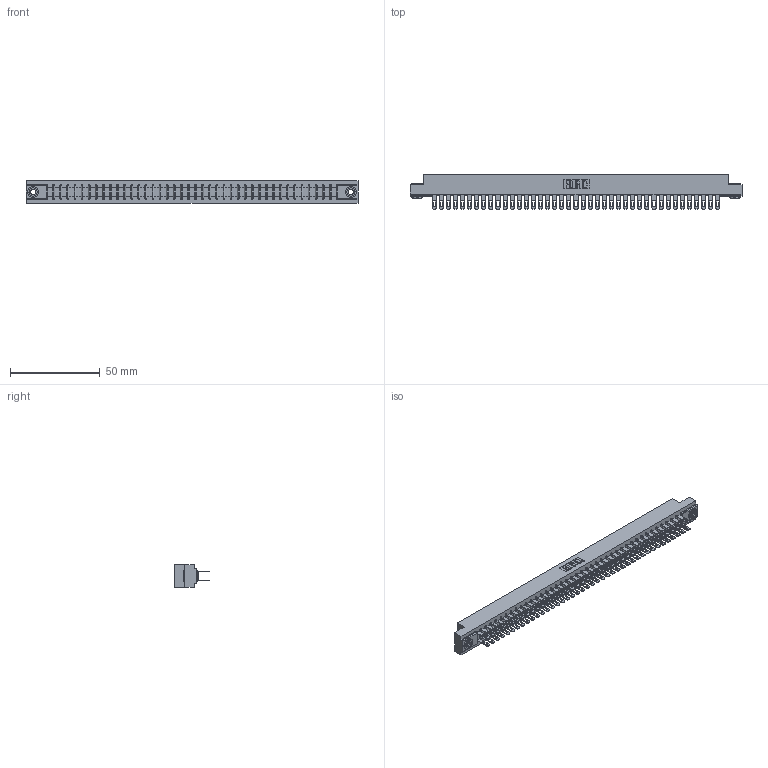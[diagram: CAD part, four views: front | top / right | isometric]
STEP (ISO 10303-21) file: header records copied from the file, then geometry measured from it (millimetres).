
FILE_DESCRIPTION (( 'STEP AP203' ), '1' );
FILE_NAME ('357-082-500-203.STEP', '2018-08-13T00:00:20', ( '' ), ( '' ), 'SwSTEP 2.0', 'SolidWorks 2016', '' );
FILE_SCHEMA (( 'CONFIG_CONTROL_DESIGN' ));
Length unit declared in the file: inch
Products named in the file (4): 345-250-002_345-250-002-102; 357-082-500-203; 307 Part_.156 Dia Mounting Holes; 307-290-001_500
Assembly tree (85 placements, depth 2):
  357-082-500-203
    307 Part_.156 Dia Mounting Holes
    307-290-001_500  x82
    345-250-002_345-250-002-102  x2
Bounding box: 185.47 x 19.18 x 12.7 mm (x, y, z)
Volume: 19951.8 mm3; surface area: 25947.5 mm2
Topology: 85 solids, 85 shells, 3984 faces, 11095 edges, 7170 vertices
Faces by surface type: plane 2554, cylinder 1338, sphere 84, cone 8
Entity records: 37623 total; most frequent: CARTESIAN_POINT 6134, ORIENTED_EDGE 6070, DIRECTION 6025, EDGE_CURVE 3035, VECTOR 2319, LINE 2319, VERTEX_POINT 1962, AXIS2_PLACEMENT_3D 1853
